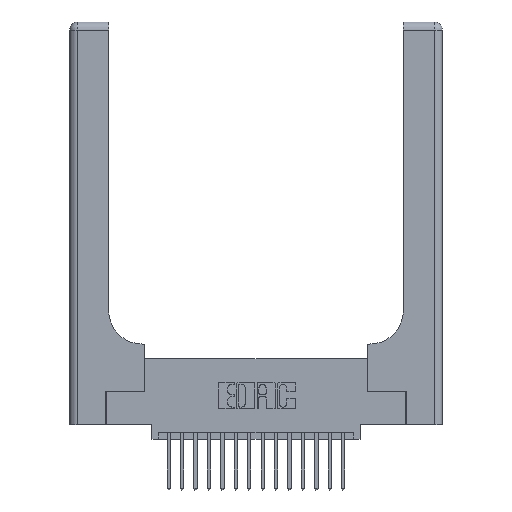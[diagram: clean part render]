
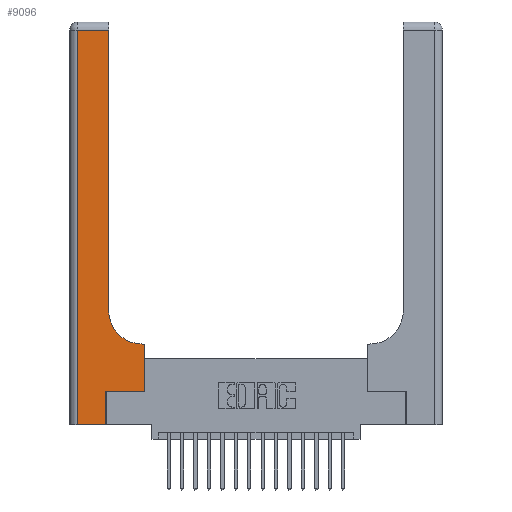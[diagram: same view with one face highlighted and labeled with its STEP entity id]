
A CAD part, top view. The second image highlights one B-rep face of the part: STEP entity #9096.
In plain terms, the highlighted planar face has unit normal (0, 0, 1).
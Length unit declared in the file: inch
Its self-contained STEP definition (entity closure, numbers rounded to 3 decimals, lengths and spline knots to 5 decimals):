
#416 = CARTESIAN_POINT ( 'NONE',  ( 0.269, 0.25, 0.37 ) ) ;
#805 = DIRECTION ( 'NONE',  ( -1., 0., 0. ) ) ;
#1311 = ORIENTED_EDGE ( 'NONE', *, *, #16918, .T. ) ;
#1615 = DIRECTION ( 'NONE',  ( 0., -1., 0. ) ) ;
#2096 = AXIS2_PLACEMENT_3D ( 'NONE', #14382, #5095, #15890 ) ;
#2401 = LINE ( 'NONE', #11162, #6239 ) ;
#2733 = VECTOR ( 'NONE', #18225, 39.37008 ) ;
#2978 = CARTESIAN_POINT ( 'NONE',  ( 0.5585, 0.25, 0.37 ) ) ;
#3080 = VECTOR ( 'NONE', #9174, 39.37008 ) ;
#3295 = LINE ( 'NONE', #5814, #8511 ) ;
#3425 = DIRECTION ( 'NONE',  ( -1., 0., 0. ) ) ;
#3776 = EDGE_CURVE ( 'NONE', #9302, #10519, #16289, .T. ) ;
#4050 = CARTESIAN_POINT ( 'NONE',  ( 0., 3., 0.37 ) ) ;
#4438 = VERTEX_POINT ( 'NONE', #18280 ) ;
#4929 = ORIENTED_EDGE ( 'NONE', *, *, #14858, .T. ) ;
#5095 = DIRECTION ( 'NONE',  ( 0., 0., -1. ) ) ;
#5271 = EDGE_CURVE ( 'NONE', #9360, #12702, #14438, .T. ) ;
#5351 = CIRCLE ( 'NONE', #2096, 0.25 ) ;
#5726 = EDGE_CURVE ( 'NONE', #10519, #4438, #2401, .T. ) ;
#5814 = CARTESIAN_POINT ( 'NONE',  ( 0.269, 0., 0.37 ) ) ;
#6183 = CARTESIAN_POINT ( 'NONE',  ( 0.2915, 2.94, 0.37 ) ) ;
#6239 = VECTOR ( 'NONE', #1615, 39.37008 ) ;
#6473 = CARTESIAN_POINT ( 'NONE',  ( 0.5415, 0.6, 0.37 ) ) ;
#6545 = VERTEX_POINT ( 'NONE', #416 ) ;
#6963 = EDGE_LOOP ( 'NONE', ( #14719, #16178, #15760, #4929, #14855, #16277, #19771, #7604, #1311 ) ) ;
#7059 = LINE ( 'NONE', #10681, #2733 ) ;
#7604 = ORIENTED_EDGE ( 'NONE', *, *, #5271, .T. ) ;
#7620 = CARTESIAN_POINT ( 'NONE',  ( 0.2915, 3., 0.37 ) ) ;
#8511 = VECTOR ( 'NONE', #19419, 39.37008 ) ;
#8527 = EDGE_CURVE ( 'NONE', #17126, #9302, #19440, .T. ) ;
#8590 = CARTESIAN_POINT ( 'NONE',  ( 0., 0., 0.37 ) ) ;
#9096 = ADVANCED_FACE ( 'NONE', ( #14089 ), #14930, .F. ) ;
#9174 = DIRECTION ( 'NONE',  ( 0., 1., 0. ) ) ;
#9302 = VERTEX_POINT ( 'NONE', #6183 ) ;
#9315 = LINE ( 'NONE', #2978, #13861 ) ;
#9360 = VERTEX_POINT ( 'NONE', #18470 ) ;
#10353 = CARTESIAN_POINT ( 'NONE',  ( 0., 2.94, 0.37 ) ) ;
#10415 = DIRECTION ( 'NONE',  ( 0., 0., -1. ) ) ;
#10519 = VERTEX_POINT ( 'NONE', #11965 ) ;
#10526 = DIRECTION ( 'NONE',  ( -1., 0., 0. ) ) ;
#10681 = CARTESIAN_POINT ( 'NONE',  ( 0.269, 0.25, 0.37 ) ) ;
#11107 = EDGE_CURVE ( 'NONE', #13216, #6545, #3295, .T. ) ;
#11162 = CARTESIAN_POINT ( 'NONE',  ( 0.06, 3., 0.37 ) ) ;
#11965 = CARTESIAN_POINT ( 'NONE',  ( 0.06, 2.94, 0.37 ) ) ;
#12050 = LINE ( 'NONE', #8590, #15571 ) ;
#12702 = VERTEX_POINT ( 'NONE', #6473 ) ;
#13216 = VERTEX_POINT ( 'NONE', #18410 ) ;
#13861 = VECTOR ( 'NONE', #13952, 39.37008 ) ;
#13952 = DIRECTION ( 'NONE',  ( 0., 1., 0. ) ) ;
#13966 = VECTOR ( 'NONE', #3425, 39.37008 ) ;
#14089 = FACE_OUTER_BOUND ( 'NONE', #6963, .T. ) ;
#14382 = CARTESIAN_POINT ( 'NONE',  ( 0.5415, 0.85, 0.37 ) ) ;
#14438 = LINE ( 'NONE', #18763, #13966 ) ;
#14719 = ORIENTED_EDGE ( 'NONE', *, *, #8527, .T. ) ;
#14851 = CARTESIAN_POINT ( 'NONE',  ( 0.2915, 0.85, 0.37 ) ) ;
#14855 = ORIENTED_EDGE ( 'NONE', *, *, #11107, .T. ) ;
#14858 = EDGE_CURVE ( 'NONE', #4438, #13216, #12050, .T. ) ;
#14930 = PLANE ( 'NONE',  #16374 ) ;
#15571 = VECTOR ( 'NONE', #16286, 39.37008 ) ;
#15760 = ORIENTED_EDGE ( 'NONE', *, *, #5726, .T. ) ;
#15890 = DIRECTION ( 'NONE',  ( 1., 0., 0. ) ) ;
#16139 = EDGE_CURVE ( 'NONE', #18469, #9360, #9315, .T. ) ;
#16178 = ORIENTED_EDGE ( 'NONE', *, *, #3776, .T. ) ;
#16277 = ORIENTED_EDGE ( 'NONE', *, *, #18952, .T. ) ;
#16286 = DIRECTION ( 'NONE',  ( 1., 0., 0. ) ) ;
#16289 = LINE ( 'NONE', #10353, #19732 ) ;
#16374 = AXIS2_PLACEMENT_3D ( 'NONE', #4050, #10415, #805 ) ;
#16918 = EDGE_CURVE ( 'NONE', #12702, #17126, #5351, .T. ) ;
#17126 = VERTEX_POINT ( 'NONE', #14851 ) ;
#18225 = DIRECTION ( 'NONE',  ( 1., 0., 0. ) ) ;
#18280 = CARTESIAN_POINT ( 'NONE',  ( 0.06, 0., 0.37 ) ) ;
#18366 = CARTESIAN_POINT ( 'NONE',  ( 0.5585, 0.25, 0.37 ) ) ;
#18410 = CARTESIAN_POINT ( 'NONE',  ( 0.269, 0., 0.37 ) ) ;
#18469 = VERTEX_POINT ( 'NONE', #18366 ) ;
#18470 = CARTESIAN_POINT ( 'NONE',  ( 0.5585, 0.6, 0.37 ) ) ;
#18763 = CARTESIAN_POINT ( 'NONE',  ( 0.2915, 0.6, 0.37 ) ) ;
#18952 = EDGE_CURVE ( 'NONE', #6545, #18469, #7059, .T. ) ;
#19419 = DIRECTION ( 'NONE',  ( 0., 1., 0. ) ) ;
#19440 = LINE ( 'NONE', #7620, #3080 ) ;
#19732 = VECTOR ( 'NONE', #10526, 39.37008 ) ;
#19771 = ORIENTED_EDGE ( 'NONE', *, *, #16139, .T. ) ;
